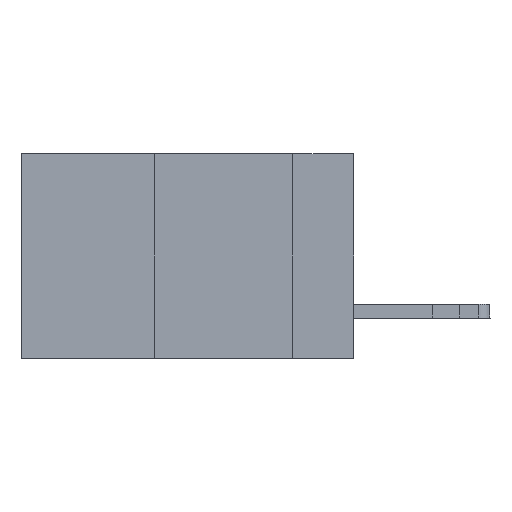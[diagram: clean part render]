
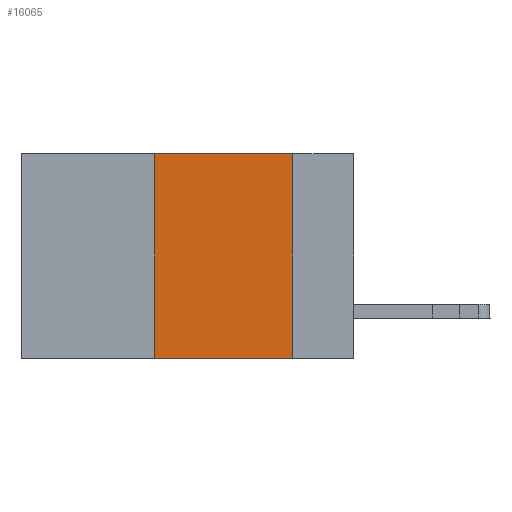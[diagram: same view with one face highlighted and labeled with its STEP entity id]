
A CAD part, left-side view. The second image highlights one B-rep face of the part: STEP entity #16065.
In plain terms, the highlighted planar face has unit normal (-1, 0, 0).
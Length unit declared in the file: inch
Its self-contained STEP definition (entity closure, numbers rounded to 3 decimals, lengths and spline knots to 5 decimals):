
#1161 = EDGE_CURVE ( 'NONE', #6306, #5434, #18641, .T. ) ;
#1304 = ORIENTED_EDGE ( 'NONE', *, *, #7326, .F. ) ;
#1430 = CARTESIAN_POINT ( 'NONE',  ( 0., 0.11, 0. ) ) ;
#1670 = DIRECTION ( 'NONE',  ( 0., 0., -1. ) ) ;
#2493 = VECTOR ( 'NONE', #12562, 39.37008 ) ;
#4332 = VECTOR ( 'NONE', #1670, 39.37008 ) ;
#5434 = VERTEX_POINT ( 'NONE', #22946 ) ;
#5625 = LINE ( 'NONE', #13674, #4332 ) ;
#5627 = AXIS2_PLACEMENT_3D ( 'NONE', #24925, #18830, #16840 ) ;
#6155 = ORIENTED_EDGE ( 'NONE', *, *, #8086, .T. ) ;
#6306 = VERTEX_POINT ( 'NONE', #22852 ) ;
#7326 = EDGE_CURVE ( 'NONE', #16213, #17631, #5625, .T. ) ;
#7889 = DIRECTION ( 'NONE',  ( 0., -1., 0. ) ) ;
#8006 = VECTOR ( 'NONE', #7889, 39.37008 ) ;
#8086 = EDGE_CURVE ( 'NONE', #6306, #17631, #23099, .T. ) ;
#10840 = FACE_OUTER_BOUND ( 'NONE', #13855, .T. ) ;
#10855 = VECTOR ( 'NONE', #21159, 39.37008 ) ;
#12562 = DIRECTION ( 'NONE',  ( 0., -1., 0. ) ) ;
#12619 = ORIENTED_EDGE ( 'NONE', *, *, #1161, .F. ) ;
#12790 = PLANE ( 'NONE',  #5627 ) ;
#13055 = ORIENTED_EDGE ( 'NONE', *, *, #24053, .F. ) ;
#13674 = CARTESIAN_POINT ( 'NONE',  ( 0., 0.11, 0. ) ) ;
#13855 = EDGE_LOOP ( 'NONE', ( #1304, #13055, #12619, #6155 ) ) ;
#16065 = ADVANCED_FACE ( 'NONE', ( #10840 ), #12790, .F. ) ;
#16213 = VERTEX_POINT ( 'NONE', #1430 ) ;
#16840 = DIRECTION ( 'NONE',  ( 0., 0., -1. ) ) ;
#17631 = VERTEX_POINT ( 'NONE', #23433 ) ;
#18641 = LINE ( 'NONE', #21031, #10855 ) ;
#18830 = DIRECTION ( 'NONE',  ( 1., 0., 0. ) ) ;
#19735 = LINE ( 'NONE', #21866, #8006 ) ;
#21031 = CARTESIAN_POINT ( 'NONE',  ( 0., 0.36, 0. ) ) ;
#21159 = DIRECTION ( 'NONE',  ( 0., 0., 1. ) ) ;
#21866 = CARTESIAN_POINT ( 'NONE',  ( 0., 0.6, 0. ) ) ;
#22852 = CARTESIAN_POINT ( 'NONE',  ( 0., 0.36, -0.37 ) ) ;
#22946 = CARTESIAN_POINT ( 'NONE',  ( 0., 0.36, 0. ) ) ;
#23099 = LINE ( 'NONE', #23231, #2493 ) ;
#23231 = CARTESIAN_POINT ( 'NONE',  ( 0., 0.6, -0.37 ) ) ;
#23433 = CARTESIAN_POINT ( 'NONE',  ( 0., 0.11, -0.37 ) ) ;
#24053 = EDGE_CURVE ( 'NONE', #5434, #16213, #19735, .T. ) ;
#24925 = CARTESIAN_POINT ( 'NONE',  ( 0., 0.6, 0. ) ) ;
